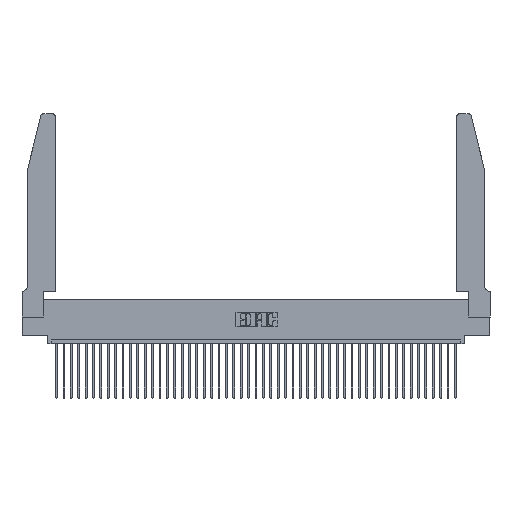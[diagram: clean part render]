
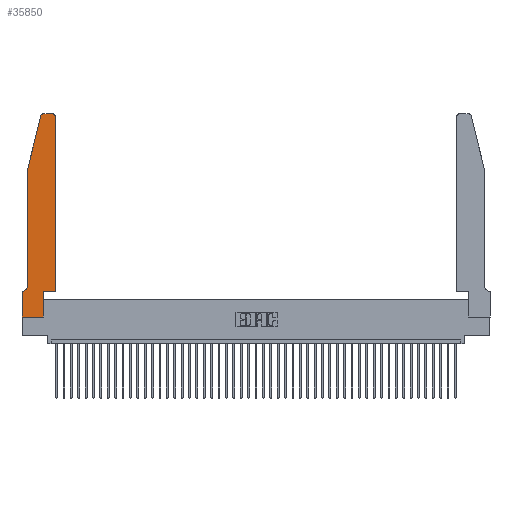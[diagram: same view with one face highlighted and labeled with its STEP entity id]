
A CAD part, top view. The second image highlights one B-rep face of the part: STEP entity #35850.
In plain terms, the highlighted planar face has unit normal (0, 0, 1).
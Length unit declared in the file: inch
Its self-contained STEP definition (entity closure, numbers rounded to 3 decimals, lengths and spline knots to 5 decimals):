
#619 = DIRECTION ( 'NONE',  ( -1., 0., 0. ) ) ;
#779 = CARTESIAN_POINT ( 'NONE',  ( 0.2605, 2.75, 0.37 ) ) ;
#1319 = ORIENTED_EDGE ( 'NONE', *, *, #35261, .T. ) ;
#1850 = EDGE_CURVE ( 'NONE', #31901, #10533, #16660, .T. ) ;
#2303 = CARTESIAN_POINT ( 'NONE',  ( 0.2865, 0., 0.37 ) ) ;
#3012 = CARTESIAN_POINT ( 'NONE',  ( 0.4505, 0.35, 0.37 ) ) ;
#3013 = DIRECTION ( 'NONE',  ( 0., 0., -1. ) ) ;
#4109 = DIRECTION ( 'NONE',  ( 1., 0., 0. ) ) ;
#4151 = VECTOR ( 'NONE', #7292, 39.37008 ) ;
#4253 = DIRECTION ( 'NONE',  ( 0., 0., 1. ) ) ;
#4674 = ORIENTED_EDGE ( 'NONE', *, *, #40958, .T. ) ;
#4677 = LINE ( 'NONE', #8964, #9637 ) ;
#4692 = CARTESIAN_POINT ( 'NONE',  ( 0., 0., 0.37 ) ) ;
#5971 = VERTEX_POINT ( 'NONE', #40604 ) ;
#5984 = ORIENTED_EDGE ( 'NONE', *, *, #40326, .T. ) ;
#6029 = DIRECTION ( 'NONE',  ( 0., 1., 0. ) ) ;
#6076 = CARTESIAN_POINT ( 'NONE',  ( 0.0055, 0.42, 0.37 ) ) ;
#6383 = DIRECTION ( 'NONE',  ( -1., 0., 0. ) ) ;
#6465 = AXIS2_PLACEMENT_3D ( 'NONE', #38928, #17768, #11347 ) ;
#6506 = DIRECTION ( 'NONE',  ( 0., 0., 1. ) ) ;
#7010 = VERTEX_POINT ( 'NONE', #34174 ) ;
#7212 = EDGE_CURVE ( 'NONE', #27991, #7010, #14441, .T. ) ;
#7292 = DIRECTION ( 'NONE',  ( 0., -1., 0. ) ) ;
#8316 = VERTEX_POINT ( 'NONE', #12882 ) ;
#8384 = DIRECTION ( 'NONE',  ( 1., 0., 0. ) ) ;
#8446 = CARTESIAN_POINT ( 'NONE',  ( 0.0055, 0.35, 0.37 ) ) ;
#8888 = AXIS2_PLACEMENT_3D ( 'NONE', #6076, #3013, #6383 ) ;
#8964 = CARTESIAN_POINT ( 'NONE',  ( 0.4505, 0.35, 0.37 ) ) ;
#9065 = VERTEX_POINT ( 'NONE', #4692 ) ;
#9418 = CARTESIAN_POINT ( 'NONE',  ( 0.4505, 0.35, 0.37 ) ) ;
#9610 = VERTEX_POINT ( 'NONE', #28340 ) ;
#9637 = VECTOR ( 'NONE', #17013, 39.37008 ) ;
#9684 = VECTOR ( 'NONE', #619, 39.37008 ) ;
#10435 = CARTESIAN_POINT ( 'NONE',  ( 0.2865, 0.35, 0.37 ) ) ;
#10533 = VERTEX_POINT ( 'NONE', #10435 ) ;
#11100 = ORIENTED_EDGE ( 'NONE', *, *, #29104, .T. ) ;
#11223 = ORIENTED_EDGE ( 'NONE', *, *, #43344, .T. ) ;
#11347 = DIRECTION ( 'NONE',  ( 1., 0., 0. ) ) ;
#11770 = LINE ( 'NONE', #779, #9684 ) ;
#12882 = CARTESIAN_POINT ( 'NONE',  ( 0., 0.35, 0.37 ) ) ;
#13331 = VERTEX_POINT ( 'NONE', #8446 ) ;
#13337 = ORIENTED_EDGE ( 'NONE', *, *, #7212, .T. ) ;
#14337 = CARTESIAN_POINT ( 'NONE',  ( 0.25487, 2.72718, 0.37 ) ) ;
#14441 = LINE ( 'NONE', #9418, #41341 ) ;
#15134 = VECTOR ( 'NONE', #8384, 39.37008 ) ;
#15406 = CIRCLE ( 'NONE', #21043, 0.03 ) ;
#16380 = DIRECTION ( 'NONE',  ( -1., 0., 0. ) ) ;
#16660 = LINE ( 'NONE', #23101, #26268 ) ;
#16921 = ORIENTED_EDGE ( 'NONE', *, *, #31757, .T. ) ;
#17013 = DIRECTION ( 'NONE',  ( 1., 0., 0. ) ) ;
#17677 = CARTESIAN_POINT ( 'NONE',  ( 0.4205, 2.72, 0.37 ) ) ;
#17768 = DIRECTION ( 'NONE',  ( 0., 0., 1. ) ) ;
#19010 = ORIENTED_EDGE ( 'NONE', *, *, #1850, .T. ) ;
#19106 = CIRCLE ( 'NONE', #6465, 0.03 ) ;
#19570 = VERTEX_POINT ( 'NONE', #39615 ) ;
#20349 = LINE ( 'NONE', #22451, #4151 ) ;
#20785 = FACE_OUTER_BOUND ( 'NONE', #32861, .T. ) ;
#21043 = AXIS2_PLACEMENT_3D ( 'NONE', #17677, #4253, #4109 ) ;
#22121 = LINE ( 'NONE', #25443, #15134 ) ;
#22451 = CARTESIAN_POINT ( 'NONE',  ( 0., 0., 0.37 ) ) ;
#23101 = CARTESIAN_POINT ( 'NONE',  ( 0.2865, 0.35, 0.37 ) ) ;
#24524 = ORIENTED_EDGE ( 'NONE', *, *, #35555, .T. ) ;
#25012 = EDGE_CURVE ( 'NONE', #19570, #13331, #40911, .T. ) ;
#25443 = CARTESIAN_POINT ( 'NONE',  ( 0., 0., 0.37 ) ) ;
#25847 = CARTESIAN_POINT ( 'NONE',  ( 0.0755, 2., 0.37 ) ) ;
#25981 = DIRECTION ( 'NONE',  ( -0.239, -0.971, 0. ) ) ;
#26268 = VECTOR ( 'NONE', #6029, 39.37008 ) ;
#26586 = EDGE_CURVE ( 'NONE', #9610, #5971, #11770, .T. ) ;
#26750 = DIRECTION ( 'NONE',  ( 1., 0., 0. ) ) ;
#27819 = CARTESIAN_POINT ( 'NONE',  ( 0.0755, 2., 0.37 ) ) ;
#27842 = VECTOR ( 'NONE', #16380, 39.37008 ) ;
#27988 = VECTOR ( 'NONE', #25981, 39.37008 ) ;
#27991 = VERTEX_POINT ( 'NONE', #3012 ) ;
#28340 = CARTESIAN_POINT ( 'NONE',  ( 0.4205, 2.75, 0.37 ) ) ;
#28563 = ORIENTED_EDGE ( 'NONE', *, *, #26586, .T. ) ;
#29034 = EDGE_CURVE ( 'NONE', #9065, #31901, #22121, .T. ) ;
#29104 = EDGE_CURVE ( 'NONE', #32910, #35167, #37183, .T. ) ;
#29556 = ORIENTED_EDGE ( 'NONE', *, *, #25012, .T. ) ;
#29744 = DIRECTION ( 'NONE',  ( 0., 1., 0. ) ) ;
#30748 = CARTESIAN_POINT ( 'NONE',  ( 0., 0.35, 0.37 ) ) ;
#31757 = EDGE_CURVE ( 'NONE', #7010, #9610, #15406, .T. ) ;
#31901 = VERTEX_POINT ( 'NONE', #2303 ) ;
#32721 = LINE ( 'NONE', #27819, #43567 ) ;
#32861 = EDGE_LOOP ( 'NONE', ( #28563, #11223, #11100, #5984, #29556, #4674, #1319, #36996, #19010, #24524, #13337, #16921 ) ) ;
#32910 = VERTEX_POINT ( 'NONE', #14337 ) ;
#33788 = PLANE ( 'NONE',  #36112 ) ;
#34174 = CARTESIAN_POINT ( 'NONE',  ( 0.4505, 2.72, 0.37 ) ) ;
#35167 = VERTEX_POINT ( 'NONE', #43514 ) ;
#35261 = EDGE_CURVE ( 'NONE', #8316, #9065, #20349, .T. ) ;
#35317 = DIRECTION ( 'NONE',  ( 0., -1., 0. ) ) ;
#35555 = EDGE_CURVE ( 'NONE', #10533, #27991, #4677, .T. ) ;
#35850 = ADVANCED_FACE ( 'NONE', ( #20785 ), #33788, .T. ) ;
#36112 = AXIS2_PLACEMENT_3D ( 'NONE', #30748, #6506, #26750 ) ;
#36637 = CARTESIAN_POINT ( 'NONE',  ( 0.0755, 0.35, 0.37 ) ) ;
#36996 = ORIENTED_EDGE ( 'NONE', *, *, #29034, .T. ) ;
#37183 = LINE ( 'NONE', #25847, #27988 ) ;
#38928 = CARTESIAN_POINT ( 'NONE',  ( 0.284, 2.72, 0.37 ) ) ;
#39615 = CARTESIAN_POINT ( 'NONE',  ( 0.0755, 0.42, 0.37 ) ) ;
#40326 = EDGE_CURVE ( 'NONE', #35167, #19570, #32721, .T. ) ;
#40348 = LINE ( 'NONE', #36637, #27842 ) ;
#40604 = CARTESIAN_POINT ( 'NONE',  ( 0.284, 2.75, 0.37 ) ) ;
#40911 = CIRCLE ( 'NONE', #8888, 0.07 ) ;
#40958 = EDGE_CURVE ( 'NONE', #13331, #8316, #40348, .T. ) ;
#41341 = VECTOR ( 'NONE', #29744, 39.37008 ) ;
#43344 = EDGE_CURVE ( 'NONE', #5971, #32910, #19106, .T. ) ;
#43514 = CARTESIAN_POINT ( 'NONE',  ( 0.0755, 2., 0.37 ) ) ;
#43567 = VECTOR ( 'NONE', #35317, 39.37008 ) ;
